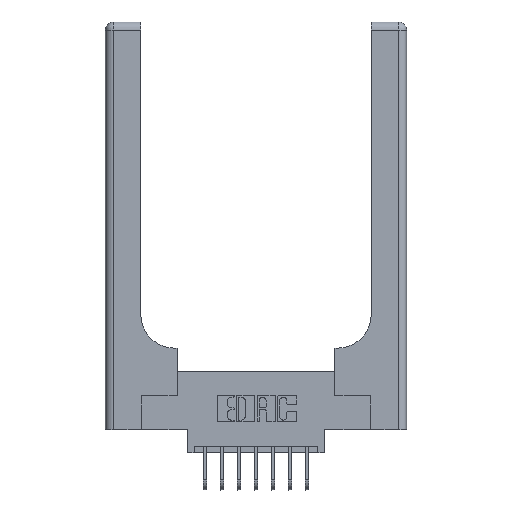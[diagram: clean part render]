
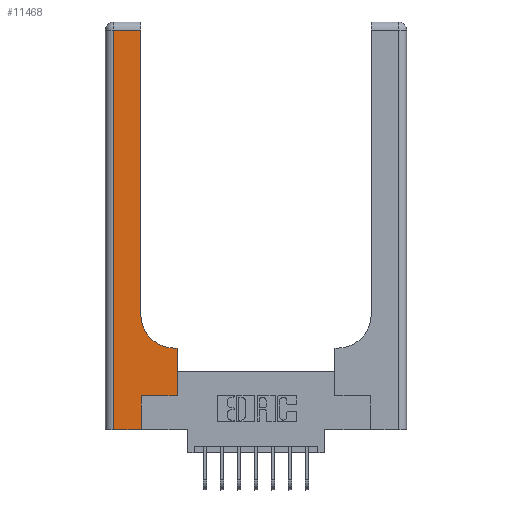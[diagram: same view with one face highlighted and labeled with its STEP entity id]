
A CAD part, top view. The second image highlights one B-rep face of the part: STEP entity #11468.
In plain terms, the highlighted planar face has unit normal (0, 0, 1).
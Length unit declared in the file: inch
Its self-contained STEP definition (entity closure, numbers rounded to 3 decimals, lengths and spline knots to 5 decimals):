
#655 = DIRECTION ( 'NONE',  ( -1., 0., 0. ) ) ;
#1355 = VERTEX_POINT ( 'NONE', #13386 ) ;
#1568 = EDGE_CURVE ( 'NONE', #3979, #5587, #15088, .T. ) ;
#1863 = DIRECTION ( 'NONE',  ( 0., -1., 0. ) ) ;
#1979 = CARTESIAN_POINT ( 'NONE',  ( 0.265, 0.25, 0.37 ) ) ;
#1980 = DIRECTION ( 'NONE',  ( 0., 1., 0. ) ) ;
#2727 = DIRECTION ( 'NONE',  ( 1., 0., 0. ) ) ;
#3979 = VERTEX_POINT ( 'NONE', #16032 ) ;
#4100 = EDGE_CURVE ( 'NONE', #10450, #15267, #15192, .T. ) ;
#4323 = VECTOR ( 'NONE', #12717, 39.37008 ) ;
#4357 = CARTESIAN_POINT ( 'NONE',  ( 0.51, 0.85, 0.37 ) ) ;
#4553 = LINE ( 'NONE', #13666, #9661 ) ;
#4721 = DIRECTION ( 'NONE',  ( 0., 1., 0. ) ) ;
#5555 = DIRECTION ( 'NONE',  ( 0., 0., -1. ) ) ;
#5577 = LINE ( 'NONE', #10993, #6289 ) ;
#5587 = VERTEX_POINT ( 'NONE', #14595 ) ;
#5667 = EDGE_CURVE ( 'NONE', #10352, #9732, #12893, .T. ) ;
#5939 = CARTESIAN_POINT ( 'NONE',  ( 0., 3., 0.37 ) ) ;
#6102 = EDGE_CURVE ( 'NONE', #5587, #10450, #15670, .T. ) ;
#6289 = VECTOR ( 'NONE', #6997, 39.37008 ) ;
#6312 = ORIENTED_EDGE ( 'NONE', *, *, #9925, .T. ) ;
#6642 = CARTESIAN_POINT ( 'NONE',  ( 0.26, 2.94, 0.37 ) ) ;
#6660 = EDGE_CURVE ( 'NONE', #9732, #8813, #4553, .T. ) ;
#6997 = DIRECTION ( 'NONE',  ( 0., 1., 0. ) ) ;
#7316 = CARTESIAN_POINT ( 'NONE',  ( 0.06, 3., 0.37 ) ) ;
#7410 = VECTOR ( 'NONE', #13920, 39.37008 ) ;
#7516 = CARTESIAN_POINT ( 'NONE',  ( 0.26, 0.6, 0.37 ) ) ;
#7542 = CARTESIAN_POINT ( 'NONE',  ( 0.26, 0.85, 0.37 ) ) ;
#7559 = ORIENTED_EDGE ( 'NONE', *, *, #4100, .T. ) ;
#7959 = VECTOR ( 'NONE', #13750, 39.37008 ) ;
#8415 = ORIENTED_EDGE ( 'NONE', *, *, #16513, .T. ) ;
#8813 = VERTEX_POINT ( 'NONE', #6642 ) ;
#9204 = CARTESIAN_POINT ( 'NONE',  ( 0., 0., 0.37 ) ) ;
#9633 = EDGE_LOOP ( 'NONE', ( #10967, #6312, #16219, #15541, #7559, #10311, #12722, #8415, #13978 ) ) ;
#9661 = VECTOR ( 'NONE', #1980, 39.37008 ) ;
#9698 = FACE_OUTER_BOUND ( 'NONE', #9633, .T. ) ;
#9732 = VERTEX_POINT ( 'NONE', #7542 ) ;
#9925 = EDGE_CURVE ( 'NONE', #8813, #3979, #15434, .T. ) ;
#10311 = ORIENTED_EDGE ( 'NONE', *, *, #13490, .T. ) ;
#10352 = VERTEX_POINT ( 'NONE', #10879 ) ;
#10450 = VERTEX_POINT ( 'NONE', #14072 ) ;
#10879 = CARTESIAN_POINT ( 'NONE',  ( 0.51, 0.6, 0.37 ) ) ;
#10944 = PLANE ( 'NONE',  #14980 ) ;
#10967 = ORIENTED_EDGE ( 'NONE', *, *, #6660, .T. ) ;
#10993 = CARTESIAN_POINT ( 'NONE',  ( 0.528, 0.25, 0.37 ) ) ;
#11031 = DIRECTION ( 'NONE',  ( 0., 0., -1. ) ) ;
#11168 = CARTESIAN_POINT ( 'NONE',  ( 0.265, 0., 0.37 ) ) ;
#11439 = LINE ( 'NONE', #7516, #4323 ) ;
#11468 = ADVANCED_FACE ( 'NONE', ( #9698 ), #10944, .F. ) ;
#12262 = EDGE_CURVE ( 'NONE', #1355, #13134, #5577, .T. ) ;
#12625 = CARTESIAN_POINT ( 'NONE',  ( 0., 2.94, 0.37 ) ) ;
#12717 = DIRECTION ( 'NONE',  ( -1., 0., 0. ) ) ;
#12722 = ORIENTED_EDGE ( 'NONE', *, *, #12262, .T. ) ;
#12893 = CIRCLE ( 'NONE', #16408, 0.25 ) ;
#13134 = VERTEX_POINT ( 'NONE', #14713 ) ;
#13175 = VECTOR ( 'NONE', #1863, 39.37008 ) ;
#13386 = CARTESIAN_POINT ( 'NONE',  ( 0.528, 0.25, 0.37 ) ) ;
#13490 = EDGE_CURVE ( 'NONE', #15267, #1355, #13667, .T. ) ;
#13578 = VECTOR ( 'NONE', #4721, 39.37008 ) ;
#13666 = CARTESIAN_POINT ( 'NONE',  ( 0.26, 3., 0.37 ) ) ;
#13667 = LINE ( 'NONE', #14696, #7959 ) ;
#13750 = DIRECTION ( 'NONE',  ( 1., 0., 0. ) ) ;
#13920 = DIRECTION ( 'NONE',  ( -1., 0., 0. ) ) ;
#13978 = ORIENTED_EDGE ( 'NONE', *, *, #5667, .T. ) ;
#14072 = CARTESIAN_POINT ( 'NONE',  ( 0.265, 0., 0.37 ) ) ;
#14527 = VECTOR ( 'NONE', #2727, 39.37008 ) ;
#14595 = CARTESIAN_POINT ( 'NONE',  ( 0.06, 0., 0.37 ) ) ;
#14696 = CARTESIAN_POINT ( 'NONE',  ( 0.265, 0.25, 0.37 ) ) ;
#14713 = CARTESIAN_POINT ( 'NONE',  ( 0.528, 0.6, 0.37 ) ) ;
#14980 = AXIS2_PLACEMENT_3D ( 'NONE', #5939, #11031, #655 ) ;
#15088 = LINE ( 'NONE', #7316, #13175 ) ;
#15192 = LINE ( 'NONE', #11168, #13578 ) ;
#15267 = VERTEX_POINT ( 'NONE', #1979 ) ;
#15434 = LINE ( 'NONE', #12625, #7410 ) ;
#15541 = ORIENTED_EDGE ( 'NONE', *, *, #6102, .T. ) ;
#15670 = LINE ( 'NONE', #9204, #14527 ) ;
#16032 = CARTESIAN_POINT ( 'NONE',  ( 0.06, 2.94, 0.37 ) ) ;
#16100 = DIRECTION ( 'NONE',  ( 1., 0., 0. ) ) ;
#16219 = ORIENTED_EDGE ( 'NONE', *, *, #1568, .T. ) ;
#16408 = AXIS2_PLACEMENT_3D ( 'NONE', #4357, #5555, #16100 ) ;
#16513 = EDGE_CURVE ( 'NONE', #13134, #10352, #11439, .T. ) ;
